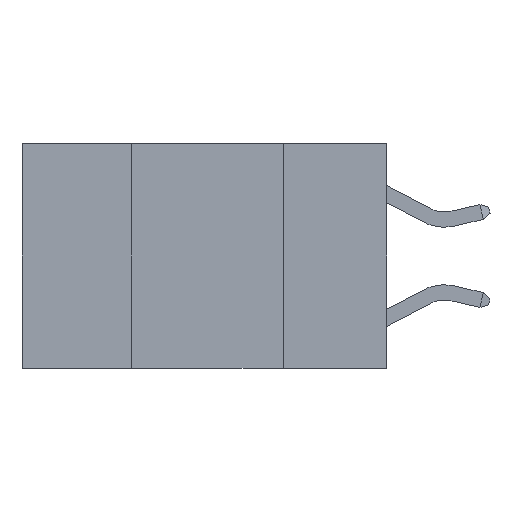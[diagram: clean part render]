
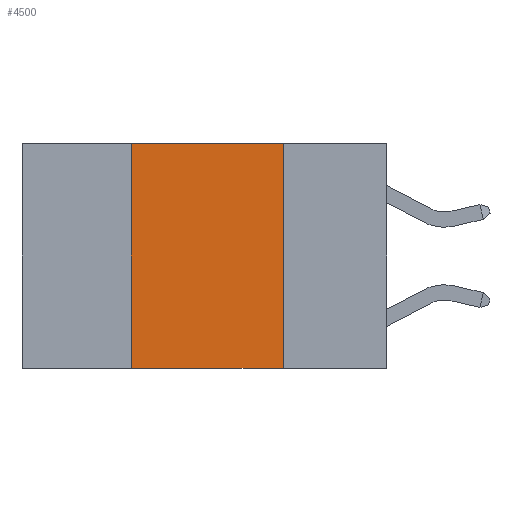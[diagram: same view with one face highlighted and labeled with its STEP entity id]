
A CAD part, left-side view. The second image highlights one B-rep face of the part: STEP entity #4500.
In plain terms, the highlighted planar face has unit normal (-1, 0, 0).
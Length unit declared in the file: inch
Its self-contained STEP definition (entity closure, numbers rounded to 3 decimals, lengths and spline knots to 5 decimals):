
#247 = CARTESIAN_POINT ( 'NONE',  ( 0., 0.6, -0.37 ) ) ;
#932 = CARTESIAN_POINT ( 'NONE',  ( 0., 0.17, -0.37 ) ) ;
#1173 = VECTOR ( 'NONE', #8282, 39.37008 ) ;
#1523 = EDGE_CURVE ( 'NONE', #7636, #4998, #5904, .T. ) ;
#1556 = LINE ( 'NONE', #8209, #1173 ) ;
#1571 = FACE_OUTER_BOUND ( 'NONE', #5444, .T. ) ;
#2070 = DIRECTION ( 'NONE',  ( 0., -1., 0. ) ) ;
#2706 = VERTEX_POINT ( 'NONE', #8001 ) ;
#2731 = AXIS2_PLACEMENT_3D ( 'NONE', #6234, #6200, #6191 ) ;
#2859 = CARTESIAN_POINT ( 'NONE',  ( 0., 0.42, 0. ) ) ;
#2934 = VERTEX_POINT ( 'NONE', #6365 ) ;
#4377 = EDGE_CURVE ( 'NONE', #2934, #4998, #1556, .T. ) ;
#4436 = ORIENTED_EDGE ( 'NONE', *, *, #4377, .F. ) ;
#4460 = ORIENTED_EDGE ( 'NONE', *, *, #9469, .F. ) ;
#4500 = ADVANCED_FACE ( 'NONE', ( #1571 ), #6427, .F. ) ;
#4521 = ORIENTED_EDGE ( 'NONE', *, *, #7275, .F. ) ;
#4558 = ORIENTED_EDGE ( 'NONE', *, *, #1523, .T. ) ;
#4998 = VERTEX_POINT ( 'NONE', #932 ) ;
#5125 = VECTOR ( 'NONE', #6479, 39.37008 ) ;
#5444 = EDGE_LOOP ( 'NONE', ( #4436, #4460, #4521, #4558 ) ) ;
#5904 = LINE ( 'NONE', #247, #6131 ) ;
#6131 = VECTOR ( 'NONE', #2070, 39.37008 ) ;
#6191 = DIRECTION ( 'NONE',  ( 0., 0., -1. ) ) ;
#6200 = DIRECTION ( 'NONE',  ( 1., 0., 0. ) ) ;
#6234 = CARTESIAN_POINT ( 'NONE',  ( 0., 0.6, 0. ) ) ;
#6365 = CARTESIAN_POINT ( 'NONE',  ( 0., 0.17, 0. ) ) ;
#6427 = PLANE ( 'NONE',  #2731 ) ;
#6479 = DIRECTION ( 'NONE',  ( 0., -1., 0. ) ) ;
#7021 = LINE ( 'NONE', #2859, #9714 ) ;
#7115 = LINE ( 'NONE', #8686, #5125 ) ;
#7275 = EDGE_CURVE ( 'NONE', #7636, #2706, #7021, .T. ) ;
#7426 = DIRECTION ( 'NONE',  ( 0., 0., 1. ) ) ;
#7636 = VERTEX_POINT ( 'NONE', #8554 ) ;
#8001 = CARTESIAN_POINT ( 'NONE',  ( 0., 0.42, 0. ) ) ;
#8209 = CARTESIAN_POINT ( 'NONE',  ( 0., 0.17, 0. ) ) ;
#8282 = DIRECTION ( 'NONE',  ( 0., 0., -1. ) ) ;
#8554 = CARTESIAN_POINT ( 'NONE',  ( 0., 0.42, -0.37 ) ) ;
#8686 = CARTESIAN_POINT ( 'NONE',  ( 0., 0.6, 0. ) ) ;
#9469 = EDGE_CURVE ( 'NONE', #2706, #2934, #7115, .T. ) ;
#9714 = VECTOR ( 'NONE', #7426, 39.37008 ) ;
